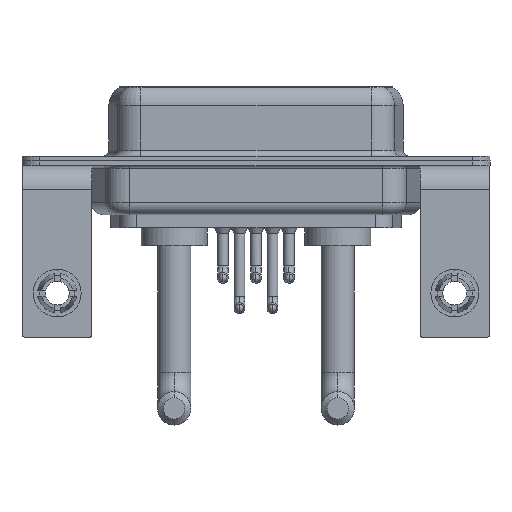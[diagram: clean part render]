
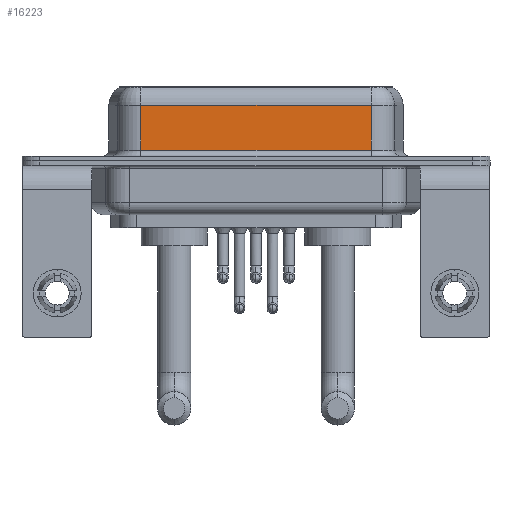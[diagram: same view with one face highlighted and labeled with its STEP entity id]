
A CAD part, front view. The second image highlights one B-rep face of the part: STEP entity #16223.
In plain terms, the highlighted planar face has unit normal (0, -1, 0).
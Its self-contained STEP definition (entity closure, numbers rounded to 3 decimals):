
#67 = CARTESIAN_POINT ( 'NONE',  ( 26.287, -3.95, 0.9 ) ) ;
#103 = LINE ( 'NONE', #4724, #840 ) ;
#298 = DIRECTION ( 'NONE',  ( 0., 0., -1. ) ) ;
#666 = EDGE_CURVE ( 'NONE', #4817, #16983, #103, .T. ) ;
#776 = LINE ( 'NONE', #6934, #10655 ) ;
#840 = VECTOR ( 'NONE', #14823, 1000. ) ;
#1563 = CARTESIAN_POINT ( 'NONE',  ( 26.287, -3.95, 0.9 ) ) ;
#2038 = EDGE_CURVE ( 'NONE', #9698, #16983, #16342, .T. ) ;
#2442 = EDGE_CURVE ( 'NONE', #3360, #9698, #18039, .T. ) ;
#2449 = DIRECTION ( 'NONE',  ( -1., 0., 0. ) ) ;
#2452 = ORIENTED_EDGE ( 'NONE', *, *, #2038, .T. ) ;
#3360 = VERTEX_POINT ( 'NONE', #12099 ) ;
#3548 = CARTESIAN_POINT ( 'NONE',  ( 7.013, -3.95, 6.4 ) ) ;
#3708 = AXIS2_PLACEMENT_3D ( 'NONE', #17106, #3777, #9701 ) ;
#3777 = DIRECTION ( 'NONE',  ( 0., 1., 0. ) ) ;
#4724 = CARTESIAN_POINT ( 'NONE',  ( 26.287, -3.95, 6.4 ) ) ;
#4817 = VERTEX_POINT ( 'NONE', #6063 ) ;
#5254 = FACE_OUTER_BOUND ( 'NONE', #17179, .T. ) ;
#6063 = CARTESIAN_POINT ( 'NONE',  ( 26.287, -3.95, 4.65 ) ) ;
#6934 = CARTESIAN_POINT ( 'NONE',  ( 26.287, -3.95, 4.65 ) ) ;
#7225 = ORIENTED_EDGE ( 'NONE', *, *, #2442, .T. ) ;
#7353 = EDGE_CURVE ( 'NONE', #4817, #3360, #776, .T. ) ;
#9698 = VERTEX_POINT ( 'NONE', #13934 ) ;
#9701 = DIRECTION ( 'NONE',  ( 0., 0., 1. ) ) ;
#10082 = ORIENTED_EDGE ( 'NONE', *, *, #666, .F. ) ;
#10310 = DIRECTION ( 'NONE',  ( 1., 0., 0. ) ) ;
#10655 = VECTOR ( 'NONE', #2449, 1000. ) ;
#11171 = PLANE ( 'NONE',  #3708 ) ;
#12099 = CARTESIAN_POINT ( 'NONE',  ( 7.013, -3.95, 4.65 ) ) ;
#13934 = CARTESIAN_POINT ( 'NONE',  ( 7.013, -3.95, 0.9 ) ) ;
#14823 = DIRECTION ( 'NONE',  ( 0., 0., -1. ) ) ;
#15269 = ORIENTED_EDGE ( 'NONE', *, *, #7353, .T. ) ;
#16223 = ADVANCED_FACE ( 'NONE', ( #5254 ), #11171, .F. ) ;
#16342 = LINE ( 'NONE', #67, #18329 ) ;
#16983 = VERTEX_POINT ( 'NONE', #1563 ) ;
#17106 = CARTESIAN_POINT ( 'NONE',  ( 26.287, -3.95, 6.4 ) ) ;
#17179 = EDGE_LOOP ( 'NONE', ( #10082, #15269, #7225, #2452 ) ) ;
#18039 = LINE ( 'NONE', #3548, #18968 ) ;
#18329 = VECTOR ( 'NONE', #10310, 1000. ) ;
#18968 = VECTOR ( 'NONE', #298, 1000. ) ;
